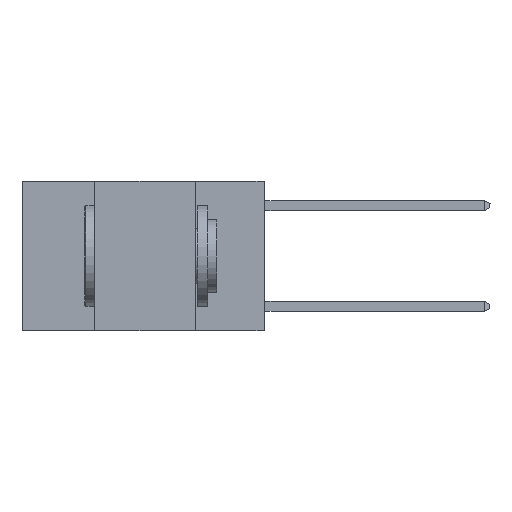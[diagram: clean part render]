
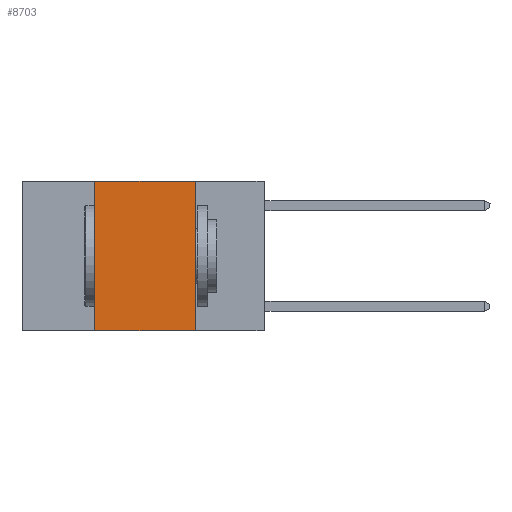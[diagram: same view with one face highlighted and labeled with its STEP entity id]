
A CAD part, left-side view. The second image highlights one B-rep face of the part: STEP entity #8703.
In plain terms, the highlighted planar face has unit normal (-1, 0, 0).
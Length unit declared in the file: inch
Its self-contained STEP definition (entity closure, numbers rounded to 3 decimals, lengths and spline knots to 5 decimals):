
#1486 = CARTESIAN_POINT ( 'NONE',  ( 0., 0.17, 0. ) ) ;
#1741 = EDGE_CURVE ( 'NONE', #7365, #20708, #14761, .T. ) ;
#2544 = DIRECTION ( 'NONE',  ( 0., -1., 0. ) ) ;
#2877 = DIRECTION ( 'NONE',  ( 0., 0., -1. ) ) ;
#3354 = DIRECTION ( 'NONE',  ( 1., 0., 0. ) ) ;
#5669 = VERTEX_POINT ( 'NONE', #29486 ) ;
#6382 = CARTESIAN_POINT ( 'NONE',  ( 0., 0.42, -0.37 ) ) ;
#6637 = ORIENTED_EDGE ( 'NONE', *, *, #1741, .T. ) ;
#6664 = LINE ( 'NONE', #31334, #13724 ) ;
#6911 = ORIENTED_EDGE ( 'NONE', *, *, #20313, .F. ) ;
#7365 = VERTEX_POINT ( 'NONE', #6382 ) ;
#8018 = EDGE_CURVE ( 'NONE', #5669, #11057, #6664, .T. ) ;
#8107 = VECTOR ( 'NONE', #23605, 39.37008 ) ;
#8703 = ADVANCED_FACE ( 'NONE', ( #18163 ), #27341, .F. ) ;
#9776 = CARTESIAN_POINT ( 'NONE',  ( 0., 0.42, 0. ) ) ;
#11057 = VERTEX_POINT ( 'NONE', #1486 ) ;
#12945 = CARTESIAN_POINT ( 'NONE',  ( 0., 0.17, -0.37 ) ) ;
#13560 = EDGE_LOOP ( 'NONE', ( #6911, #19425, #15700, #6637 ) ) ;
#13724 = VECTOR ( 'NONE', #17117, 39.37008 ) ;
#14600 = LINE ( 'NONE', #9776, #28825 ) ;
#14761 = LINE ( 'NONE', #24593, #30228 ) ;
#15570 = EDGE_CURVE ( 'NONE', #7365, #5669, #14600, .T. ) ;
#15700 = ORIENTED_EDGE ( 'NONE', *, *, #15570, .F. ) ;
#17117 = DIRECTION ( 'NONE',  ( 0., -1., 0. ) ) ;
#18163 = FACE_OUTER_BOUND ( 'NONE', #13560, .T. ) ;
#19425 = ORIENTED_EDGE ( 'NONE', *, *, #8018, .F. ) ;
#20313 = EDGE_CURVE ( 'NONE', #11057, #20708, #28751, .T. ) ;
#20708 = VERTEX_POINT ( 'NONE', #12945 ) ;
#22339 = DIRECTION ( 'NONE',  ( 0., 0., 1. ) ) ;
#22668 = CARTESIAN_POINT ( 'NONE',  ( 0., 0.6, 0. ) ) ;
#23605 = DIRECTION ( 'NONE',  ( 0., 0., -1. ) ) ;
#23761 = CARTESIAN_POINT ( 'NONE',  ( 0., 0.17, 0. ) ) ;
#24221 = AXIS2_PLACEMENT_3D ( 'NONE', #22668, #3354, #2877 ) ;
#24593 = CARTESIAN_POINT ( 'NONE',  ( 0., 0.6, -0.37 ) ) ;
#27341 = PLANE ( 'NONE',  #24221 ) ;
#28751 = LINE ( 'NONE', #23761, #8107 ) ;
#28825 = VECTOR ( 'NONE', #22339, 39.37008 ) ;
#29486 = CARTESIAN_POINT ( 'NONE',  ( 0., 0.42, 0. ) ) ;
#30228 = VECTOR ( 'NONE', #2544, 39.37008 ) ;
#31334 = CARTESIAN_POINT ( 'NONE',  ( 0., 0.6, 0. ) ) ;
